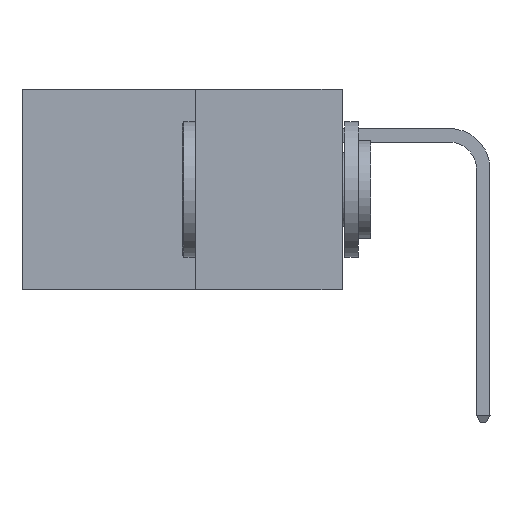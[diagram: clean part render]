
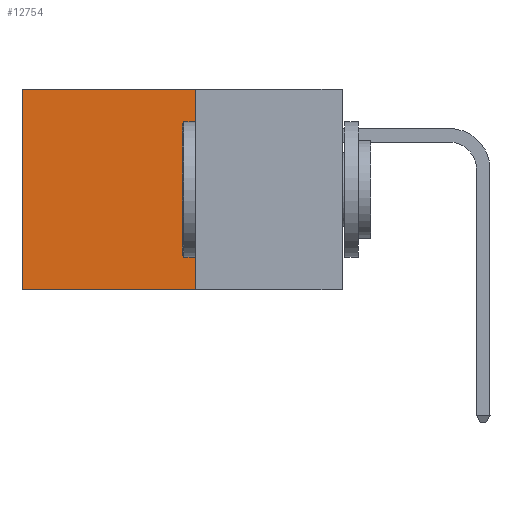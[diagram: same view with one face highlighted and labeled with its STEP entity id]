
A CAD part, left-side view. The second image highlights one B-rep face of the part: STEP entity #12754.
In plain terms, the highlighted planar face has unit normal (-1, 0, 0).
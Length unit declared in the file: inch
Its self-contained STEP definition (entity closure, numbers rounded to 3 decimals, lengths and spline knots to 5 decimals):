
#1307 = CARTESIAN_POINT ( 'NONE',  ( 0.277, 0.27, -0.37 ) ) ;
#1646 = VECTOR ( 'NONE', #29610, 39.37008 ) ;
#2125 = ORIENTED_EDGE ( 'NONE', *, *, #27417, .F. ) ;
#2127 = CARTESIAN_POINT ( 'NONE',  ( 0.277, 0.59, -0.37 ) ) ;
#2144 = ORIENTED_EDGE ( 'NONE', *, *, #4539, .T. ) ;
#2598 = EDGE_CURVE ( 'NONE', #23070, #19591, #15481, .T. ) ;
#3239 = DIRECTION ( 'NONE',  ( 0., 1., 0. ) ) ;
#4539 = EDGE_CURVE ( 'NONE', #24759, #18134, #8172, .T. ) ;
#5918 = PLANE ( 'NONE',  #15826 ) ;
#6132 = EDGE_LOOP ( 'NONE', ( #2144, #2125, #29127, #6926 ) ) ;
#6304 = DIRECTION ( 'NONE',  ( 0., 0., -1. ) ) ;
#6926 = ORIENTED_EDGE ( 'NONE', *, *, #20579, .T. ) ;
#8172 = LINE ( 'NONE', #22388, #14503 ) ;
#11787 = LINE ( 'NONE', #19684, #15820 ) ;
#12754 = ADVANCED_FACE ( 'NONE', ( #25129 ), #5918, .F. ) ;
#13153 = DIRECTION ( 'NONE',  ( 0., 0., -1. ) ) ;
#14503 = VECTOR ( 'NONE', #22229, 39.37008 ) ;
#15481 = LINE ( 'NONE', #22266, #27108 ) ;
#15820 = VECTOR ( 'NONE', #3239, 39.37008 ) ;
#15826 = AXIS2_PLACEMENT_3D ( 'NONE', #22376, #27066, #13153 ) ;
#18134 = VERTEX_POINT ( 'NONE', #2127 ) ;
#19591 = VERTEX_POINT ( 'NONE', #29863 ) ;
#19684 = CARTESIAN_POINT ( 'NONE',  ( 0.277, 0.27, 0. ) ) ;
#20579 = EDGE_CURVE ( 'NONE', #23070, #24759, #11787, .T. ) ;
#20644 = LINE ( 'NONE', #1307, #1646 ) ;
#22229 = DIRECTION ( 'NONE',  ( 0., 0., -1. ) ) ;
#22266 = CARTESIAN_POINT ( 'NONE',  ( 0.277, 0.27, -0.37 ) ) ;
#22376 = CARTESIAN_POINT ( 'NONE',  ( 0.277, 0.27, -0.37 ) ) ;
#22388 = CARTESIAN_POINT ( 'NONE',  ( 0.277, 0.59, -0.37 ) ) ;
#23070 = VERTEX_POINT ( 'NONE', #26630 ) ;
#24759 = VERTEX_POINT ( 'NONE', #27839 ) ;
#25129 = FACE_OUTER_BOUND ( 'NONE', #6132, .T. ) ;
#26630 = CARTESIAN_POINT ( 'NONE',  ( 0.277, 0.27, 0. ) ) ;
#27066 = DIRECTION ( 'NONE',  ( 1., 0., 0. ) ) ;
#27108 = VECTOR ( 'NONE', #6304, 39.37008 ) ;
#27417 = EDGE_CURVE ( 'NONE', #19591, #18134, #20644, .T. ) ;
#27839 = CARTESIAN_POINT ( 'NONE',  ( 0.277, 0.59, 0. ) ) ;
#29127 = ORIENTED_EDGE ( 'NONE', *, *, #2598, .F. ) ;
#29610 = DIRECTION ( 'NONE',  ( 0., 1., 0. ) ) ;
#29863 = CARTESIAN_POINT ( 'NONE',  ( 0.277, 0.27, -0.37 ) ) ;
